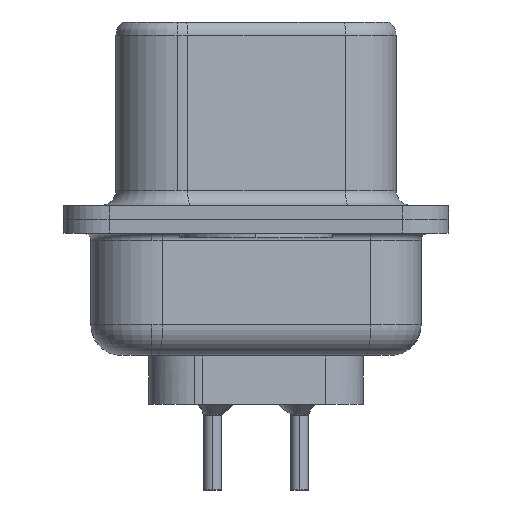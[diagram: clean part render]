
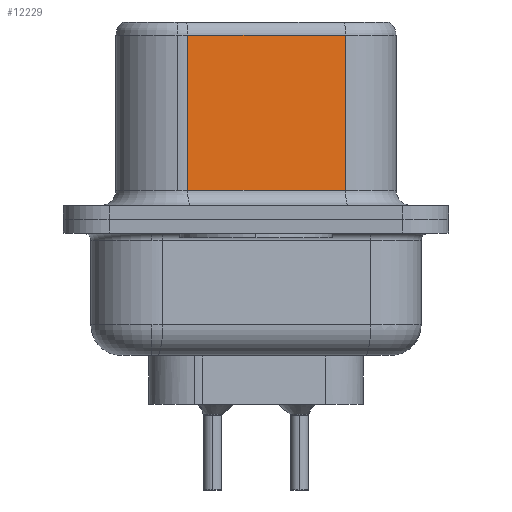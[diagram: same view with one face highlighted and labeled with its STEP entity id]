
A CAD part, left-side view. The second image highlights one B-rep face of the part: STEP entity #12229.
In plain terms, the highlighted planar face has unit normal (-0.985, -0.174, 0).
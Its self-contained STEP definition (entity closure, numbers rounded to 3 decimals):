
#325 = VECTOR ( 'NONE', #2271, 1000. ) ;
#335 = DIRECTION ( 'NONE',  ( -0.174, 0.985, 0. ) ) ;
#1382 = ORIENTED_EDGE ( 'NONE', *, *, #10652, .T. ) ;
#1628 = CARTESIAN_POINT ( 'NONE',  ( 4.575, -2.927, 6.52 ) ) ;
#1878 = VECTOR ( 'NONE', #335, 1000. ) ;
#1966 = ORIENTED_EDGE ( 'NONE', *, *, #15077, .T. ) ;
#2271 = DIRECTION ( 'NONE',  ( 0.174, -0.985, 0. ) ) ;
#2633 = DIRECTION ( 'NONE',  ( 0.985, 0.174, 0. ) ) ;
#2882 = LINE ( 'NONE', #1628, #16215 ) ;
#3012 = CARTESIAN_POINT ( 'NONE',  ( 4.575, -2.927, 6.02 ) ) ;
#3774 = VECTOR ( 'NONE', #10040, 1000. ) ;
#5206 = ORIENTED_EDGE ( 'NONE', *, *, #11751, .F. ) ;
#5554 = CARTESIAN_POINT ( 'NONE',  ( 4.575, -2.927, 6.02 ) ) ;
#7213 = LINE ( 'NONE', #13868, #3774 ) ;
#7250 = LINE ( 'NONE', #10063, #325 ) ;
#7637 = ORIENTED_EDGE ( 'NONE', *, *, #16027, .T. ) ;
#7984 = CARTESIAN_POINT ( 'NONE',  ( 3.665, 2.233, 0.95 ) ) ;
#8260 = VERTEX_POINT ( 'NONE', #3012 ) ;
#9402 = DIRECTION ( 'NONE',  ( 0., 0., -1. ) ) ;
#9951 = AXIS2_PLACEMENT_3D ( 'NONE', #15464, #2633, #11721 ) ;
#10040 = DIRECTION ( 'NONE',  ( 0., 0., -1. ) ) ;
#10063 = CARTESIAN_POINT ( 'NONE',  ( 4.575, -2.927, 0.95 ) ) ;
#10426 = PLANE ( 'NONE',  #9951 ) ;
#10582 = VERTEX_POINT ( 'NONE', #7984 ) ;
#10652 = EDGE_CURVE ( 'NONE', #8260, #14079, #15642, .T. ) ;
#11262 = VERTEX_POINT ( 'NONE', #16046 ) ;
#11721 = DIRECTION ( 'NONE',  ( -0.174, 0.985, 0. ) ) ;
#11751 = EDGE_CURVE ( 'NONE', #8260, #11262, #2882, .T. ) ;
#12229 = ADVANCED_FACE ( 'NONE', ( #16627 ), #10426, .F. ) ;
#12448 = EDGE_LOOP ( 'NONE', ( #5206, #1382, #7637, #1966 ) ) ;
#13868 = CARTESIAN_POINT ( 'NONE',  ( 3.665, 2.233, 6.52 ) ) ;
#14079 = VERTEX_POINT ( 'NONE', #15541 ) ;
#15077 = EDGE_CURVE ( 'NONE', #10582, #11262, #7250, .T. ) ;
#15464 = CARTESIAN_POINT ( 'NONE',  ( 4.575, -2.927, 6.52 ) ) ;
#15541 = CARTESIAN_POINT ( 'NONE',  ( 3.665, 2.233, 6.02 ) ) ;
#15642 = LINE ( 'NONE', #5554, #1878 ) ;
#16027 = EDGE_CURVE ( 'NONE', #14079, #10582, #7213, .T. ) ;
#16046 = CARTESIAN_POINT ( 'NONE',  ( 4.575, -2.927, 0.95 ) ) ;
#16215 = VECTOR ( 'NONE', #9402, 1000. ) ;
#16627 = FACE_OUTER_BOUND ( 'NONE', #12448, .T. ) ;
